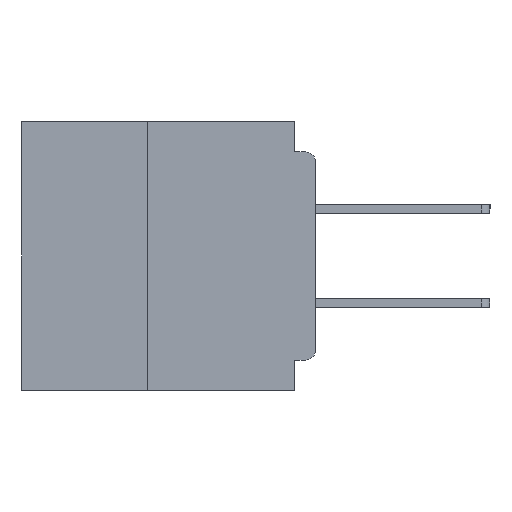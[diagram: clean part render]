
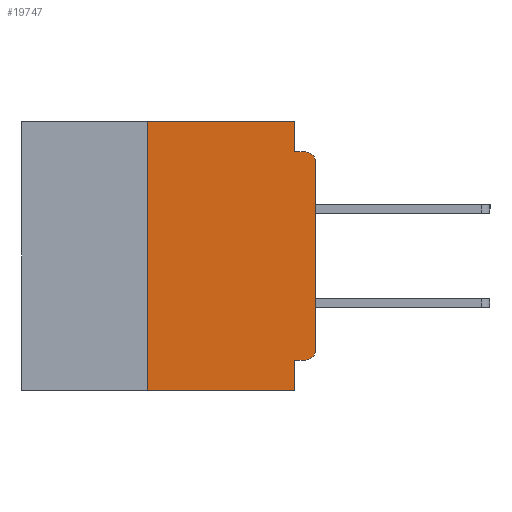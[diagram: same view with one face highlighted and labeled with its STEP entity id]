
A CAD part, left-side view. The second image highlights one B-rep face of the part: STEP entity #19747.
In plain terms, the highlighted planar face has unit normal (-1, 0, 0).
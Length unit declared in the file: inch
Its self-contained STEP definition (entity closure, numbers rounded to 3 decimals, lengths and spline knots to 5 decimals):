
#23 = CARTESIAN_POINT ( 'NONE',  ( 0., 0.25, 0. ) ) ;
#364 = CARTESIAN_POINT ( 'NONE',  ( 0., 0.437, -0.4 ) ) ;
#1107 = VERTEX_POINT ( 'NONE', #17101 ) ;
#2665 = CARTESIAN_POINT ( 'NONE',  ( 0., 0.031, -0.355 ) ) ;
#2863 = CARTESIAN_POINT ( 'NONE',  ( 0., 0., -0.06 ) ) ;
#2883 = VECTOR ( 'NONE', #35145, 39.37008 ) ;
#2943 = VERTEX_POINT ( 'NONE', #23480 ) ;
#2970 = ORIENTED_EDGE ( 'NONE', *, *, #8569, .T. ) ;
#4598 = CARTESIAN_POINT ( 'NONE',  ( 0., 0.031, -0.4 ) ) ;
#5600 = VERTEX_POINT ( 'NONE', #26181 ) ;
#6259 = DIRECTION ( 'NONE',  ( 0., 0., -1. ) ) ;
#6353 = ORIENTED_EDGE ( 'NONE', *, *, #10168, .F. ) ;
#6652 = DIRECTION ( 'NONE',  ( 0., -1., 0. ) ) ;
#7095 = CARTESIAN_POINT ( 'NONE',  ( 0., 0.015, -0.06 ) ) ;
#7432 = ORIENTED_EDGE ( 'NONE', *, *, #32225, .T. ) ;
#7978 = EDGE_LOOP ( 'NONE', ( #7432, #20007, #26986, #20146, #16868, #22985, #31633, #6353, #10119, #2970 ) ) ;
#8322 = DIRECTION ( 'NONE',  ( -1., 0., 0. ) ) ;
#8569 = EDGE_CURVE ( 'NONE', #5600, #32532, #31036, .T. ) ;
#9058 = EDGE_CURVE ( 'NONE', #38471, #13192, #29071, .T. ) ;
#9347 = CARTESIAN_POINT ( 'NONE',  ( 0., 0.031, -0.4 ) ) ;
#9960 = EDGE_CURVE ( 'NONE', #13602, #2943, #28562, .T. ) ;
#10119 = ORIENTED_EDGE ( 'NONE', *, *, #32337, .F. ) ;
#10168 = EDGE_CURVE ( 'NONE', #15137, #35937, #30000, .T. ) ;
#10219 = DIRECTION ( 'NONE',  ( 0., 0., -1. ) ) ;
#10422 = CARTESIAN_POINT ( 'NONE',  ( 0., 0.015, -0.045 ) ) ;
#10470 = CARTESIAN_POINT ( 'NONE',  ( 0., 0., -0.045 ) ) ;
#11906 = CIRCLE ( 'NONE', #35304, 0.015 ) ;
#12551 = LINE ( 'NONE', #364, #36323 ) ;
#12909 = AXIS2_PLACEMENT_3D ( 'NONE', #27762, #15436, #37055 ) ;
#13192 = VERTEX_POINT ( 'NONE', #10422 ) ;
#13602 = VERTEX_POINT ( 'NONE', #23 ) ;
#13998 = DIRECTION ( 'NONE',  ( 0., 1., 0. ) ) ;
#14023 = DIRECTION ( 'NONE',  ( 0., 0., -1. ) ) ;
#15137 = VERTEX_POINT ( 'NONE', #2665 ) ;
#15436 = DIRECTION ( 'NONE',  ( 1., 0., 0. ) ) ;
#16868 = ORIENTED_EDGE ( 'NONE', *, *, #9960, .F. ) ;
#17101 = CARTESIAN_POINT ( 'NONE',  ( 0., 0.25, -0.4 ) ) ;
#19069 = CARTESIAN_POINT ( 'NONE',  ( 0., 0.437, 0. ) ) ;
#19747 = ADVANCED_FACE ( 'NONE', ( #21371 ), #33981, .F. ) ;
#19887 = DIRECTION ( 'NONE',  ( 0., -1., 0. ) ) ;
#20007 = ORIENTED_EDGE ( 'NONE', *, *, #21997, .T. ) ;
#20146 = ORIENTED_EDGE ( 'NONE', *, *, #29141, .F. ) ;
#20331 = VECTOR ( 'NONE', #6652, 39.37008 ) ;
#20837 = VECTOR ( 'NONE', #19887, 39.37008 ) ;
#21086 = CARTESIAN_POINT ( 'NONE',  ( 0., 0., -0.34 ) ) ;
#21371 = FACE_OUTER_BOUND ( 'NONE', #7978, .T. ) ;
#21997 = EDGE_CURVE ( 'NONE', #23659, #13192, #11906, .T. ) ;
#22799 = DIRECTION ( 'NONE',  ( 0., 0., 1. ) ) ;
#22985 = ORIENTED_EDGE ( 'NONE', *, *, #36759, .F. ) ;
#23480 = CARTESIAN_POINT ( 'NONE',  ( 0., 0.031, 0. ) ) ;
#23659 = VERTEX_POINT ( 'NONE', #2863 ) ;
#24795 = LINE ( 'NONE', #32595, #33055 ) ;
#25948 = CARTESIAN_POINT ( 'NONE',  ( 0., 0.031, -0.045 ) ) ;
#26181 = CARTESIAN_POINT ( 'NONE',  ( 0., 0.015, -0.355 ) ) ;
#26963 = CARTESIAN_POINT ( 'NONE',  ( 0., 0.015, -0.34 ) ) ;
#26986 = ORIENTED_EDGE ( 'NONE', *, *, #9058, .F. ) ;
#27728 = LINE ( 'NONE', #28952, #2883 ) ;
#27762 = CARTESIAN_POINT ( 'NONE',  ( 0., 0.437, 0. ) ) ;
#28047 = VECTOR ( 'NONE', #6259, 39.37008 ) ;
#28360 = VECTOR ( 'NONE', #22799, 39.37008 ) ;
#28562 = LINE ( 'NONE', #19069, #20331 ) ;
#28859 = DIRECTION ( 'NONE',  ( -1., 0., 0. ) ) ;
#28952 = CARTESIAN_POINT ( 'NONE',  ( 0., 0., 0. ) ) ;
#29036 = VECTOR ( 'NONE', #14023, 39.37008 ) ;
#29071 = LINE ( 'NONE', #10470, #20837 ) ;
#29141 = EDGE_CURVE ( 'NONE', #2943, #38471, #36252, .T. ) ;
#30000 = LINE ( 'NONE', #4598, #29036 ) ;
#30079 = DIRECTION ( 'NONE',  ( 0., 0., -1. ) ) ;
#31036 = CIRCLE ( 'NONE', #39322, 0.015 ) ;
#31633 = ORIENTED_EDGE ( 'NONE', *, *, #40125, .T. ) ;
#32133 = CARTESIAN_POINT ( 'NONE',  ( 0., 0.25, -0.4 ) ) ;
#32225 = EDGE_CURVE ( 'NONE', #32532, #23659, #27728, .T. ) ;
#32337 = EDGE_CURVE ( 'NONE', #5600, #15137, #24795, .T. ) ;
#32532 = VERTEX_POINT ( 'NONE', #21086 ) ;
#32595 = CARTESIAN_POINT ( 'NONE',  ( 0., 0., -0.355 ) ) ;
#33055 = VECTOR ( 'NONE', #13998, 39.37008 ) ;
#33981 = PLANE ( 'NONE',  #12909 ) ;
#34477 = DIRECTION ( 'NONE',  ( 0., -1., 0. ) ) ;
#35145 = DIRECTION ( 'NONE',  ( 0., 0., 1. ) ) ;
#35304 = AXIS2_PLACEMENT_3D ( 'NONE', #7095, #28859, #10219 ) ;
#35937 = VERTEX_POINT ( 'NONE', #9347 ) ;
#36252 = LINE ( 'NONE', #37173, #28047 ) ;
#36323 = VECTOR ( 'NONE', #34477, 39.37008 ) ;
#36759 = EDGE_CURVE ( 'NONE', #1107, #13602, #37502, .T. ) ;
#37055 = DIRECTION ( 'NONE',  ( 0., 0., -1. ) ) ;
#37173 = CARTESIAN_POINT ( 'NONE',  ( 0., 0.031, 0. ) ) ;
#37502 = LINE ( 'NONE', #32133, #28360 ) ;
#38471 = VERTEX_POINT ( 'NONE', #25948 ) ;
#39322 = AXIS2_PLACEMENT_3D ( 'NONE', #26963, #8322, #30079 ) ;
#40125 = EDGE_CURVE ( 'NONE', #1107, #35937, #12551, .T. ) ;
